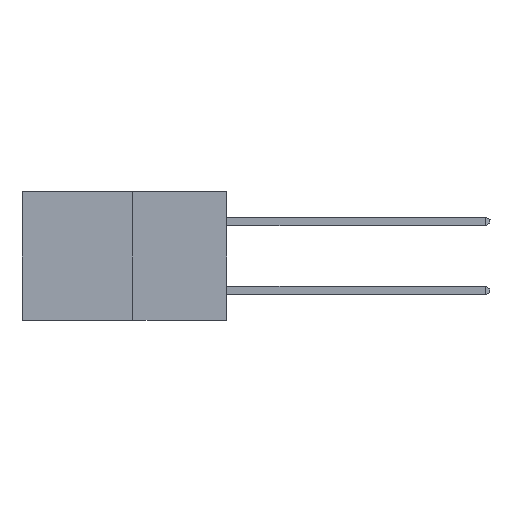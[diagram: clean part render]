
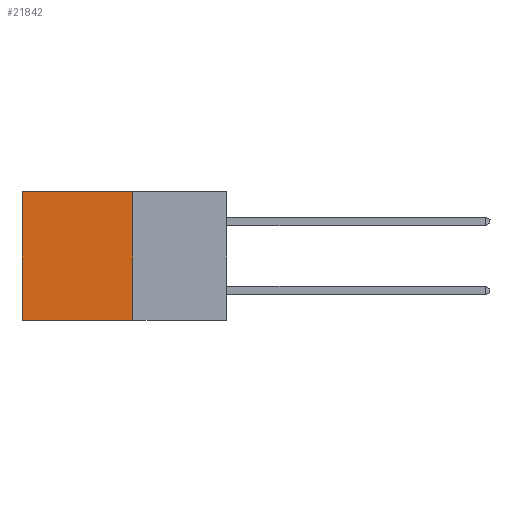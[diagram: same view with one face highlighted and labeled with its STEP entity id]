
A CAD part, left-side view. The second image highlights one B-rep face of the part: STEP entity #21842.
In plain terms, the highlighted planar face has unit normal (-1, 0, 0).
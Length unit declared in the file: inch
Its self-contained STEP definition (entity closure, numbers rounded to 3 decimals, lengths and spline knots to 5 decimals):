
#873 = CARTESIAN_POINT ( 'NONE',  ( 0.277, 0.59, -0.37 ) ) ;
#2128 = PLANE ( 'NONE',  #8761 ) ;
#2952 = CARTESIAN_POINT ( 'NONE',  ( 0.277, 0.59, 0. ) ) ;
#3096 = CARTESIAN_POINT ( 'NONE',  ( 0.277, 0.59, -0.37 ) ) ;
#4809 = VECTOR ( 'NONE', #14371, 39.37008 ) ;
#4932 = ORIENTED_EDGE ( 'NONE', *, *, #24341, .T. ) ;
#5352 = EDGE_CURVE ( 'NONE', #23904, #27105, #14186, .T. ) ;
#6222 = VERTEX_POINT ( 'NONE', #2952 ) ;
#6362 = ORIENTED_EDGE ( 'NONE', *, *, #12055, .F. ) ;
#6649 = DIRECTION ( 'NONE',  ( 1., 0., 0. ) ) ;
#7557 = DIRECTION ( 'NONE',  ( 0., 1., 0. ) ) ;
#8055 = VERTEX_POINT ( 'NONE', #3096 ) ;
#8311 = VECTOR ( 'NONE', #14366, 39.37008 ) ;
#8761 = AXIS2_PLACEMENT_3D ( 'NONE', #15660, #6649, #17752 ) ;
#10753 = EDGE_LOOP ( 'NONE', ( #4932, #6362, #17105, #23871 ) ) ;
#12055 = EDGE_CURVE ( 'NONE', #27105, #8055, #25594, .T. ) ;
#12080 = DIRECTION ( 'NONE',  ( 0., 0., -1. ) ) ;
#14186 = LINE ( 'NONE', #24092, #8311 ) ;
#14366 = DIRECTION ( 'NONE',  ( 0., 0., -1. ) ) ;
#14371 = DIRECTION ( 'NONE',  ( 0., 1., 0. ) ) ;
#14817 = VECTOR ( 'NONE', #7557, 39.37008 ) ;
#14850 = FACE_OUTER_BOUND ( 'NONE', #10753, .T. ) ;
#15660 = CARTESIAN_POINT ( 'NONE',  ( 0.277, 0.27, -0.37 ) ) ;
#16418 = EDGE_CURVE ( 'NONE', #23904, #6222, #16647, .T. ) ;
#16647 = LINE ( 'NONE', #18632, #4809 ) ;
#17105 = ORIENTED_EDGE ( 'NONE', *, *, #5352, .F. ) ;
#17752 = DIRECTION ( 'NONE',  ( 0., 0., -1. ) ) ;
#18146 = VECTOR ( 'NONE', #12080, 39.37008 ) ;
#18632 = CARTESIAN_POINT ( 'NONE',  ( 0.277, 0.27, 0. ) ) ;
#21842 = ADVANCED_FACE ( 'NONE', ( #14850 ), #2128, .F. ) ;
#23863 = LINE ( 'NONE', #873, #18146 ) ;
#23871 = ORIENTED_EDGE ( 'NONE', *, *, #16418, .T. ) ;
#23904 = VERTEX_POINT ( 'NONE', #28046 ) ;
#24092 = CARTESIAN_POINT ( 'NONE',  ( 0.277, 0.27, -0.37 ) ) ;
#24341 = EDGE_CURVE ( 'NONE', #6222, #8055, #23863, .T. ) ;
#25594 = LINE ( 'NONE', #27011, #14817 ) ;
#25627 = CARTESIAN_POINT ( 'NONE',  ( 0.277, 0.27, -0.37 ) ) ;
#27011 = CARTESIAN_POINT ( 'NONE',  ( 0.277, 0.27, -0.37 ) ) ;
#27105 = VERTEX_POINT ( 'NONE', #25627 ) ;
#28046 = CARTESIAN_POINT ( 'NONE',  ( 0.277, 0.27, 0. ) ) ;
